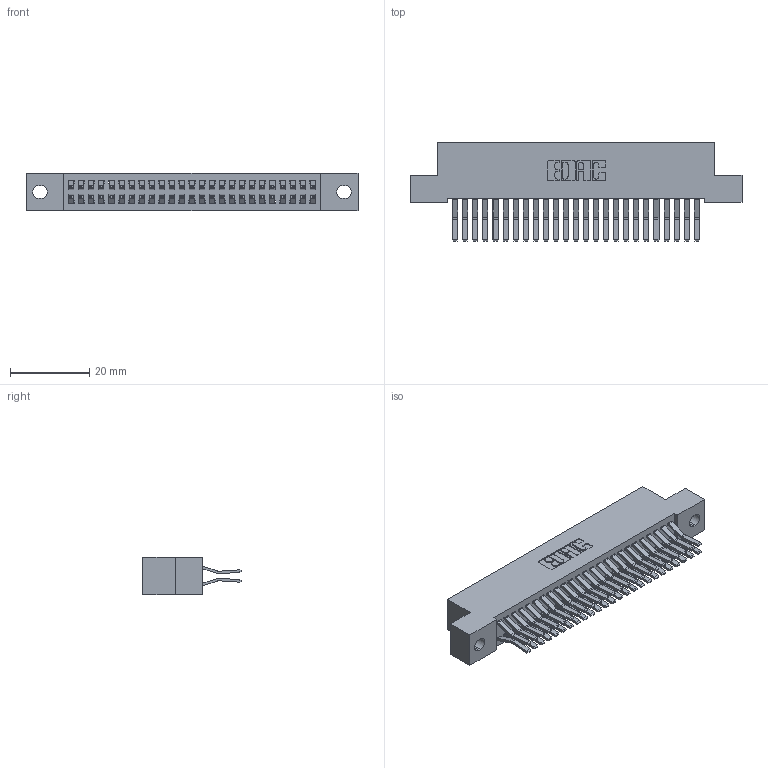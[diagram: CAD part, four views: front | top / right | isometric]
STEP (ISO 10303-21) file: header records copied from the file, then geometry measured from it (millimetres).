
FILE_DESCRIPTION (( 'STEP AP203' ), '1' );
FILE_NAME ('342-050-560-202.STEP', '2019-10-03T00:12:05', ( '' ), ( '' ), 'SwSTEP 2.0', 'SolidWorks 2016', '' );
FILE_SCHEMA (( 'CONFIG_CONTROL_DESIGN' ));
Length unit declared in the file: inch
Products named in the file (3): 342 Part_.128 Slot; 345-292-001_560 Tail; 342-050-560-202
Assembly tree (51 placements, depth 2):
  342-050-560-202
    342 Part_.128 Slot
    345-292-001_560 Tail  x50
Bounding box: 83.82 x 24.78 x 9.4 mm (x, y, z)
Volume: 7726.9 mm3; surface area: 12705.1 mm2
Topology: 51 solids, 51 shells, 2814 faces, 8361 edges, 5506 vertices
Faces by surface type: plane 1870, cylinder 944
Entity records: 18373 total; most frequent: CARTESIAN_POINT 3066, ORIENTED_EDGE 3002, DIRECTION 2653, EDGE_CURVE 1501, VECTOR 1369, LINE 1369, VERTEX_POINT 998, AXIS2_PLACEMENT_3D 642
